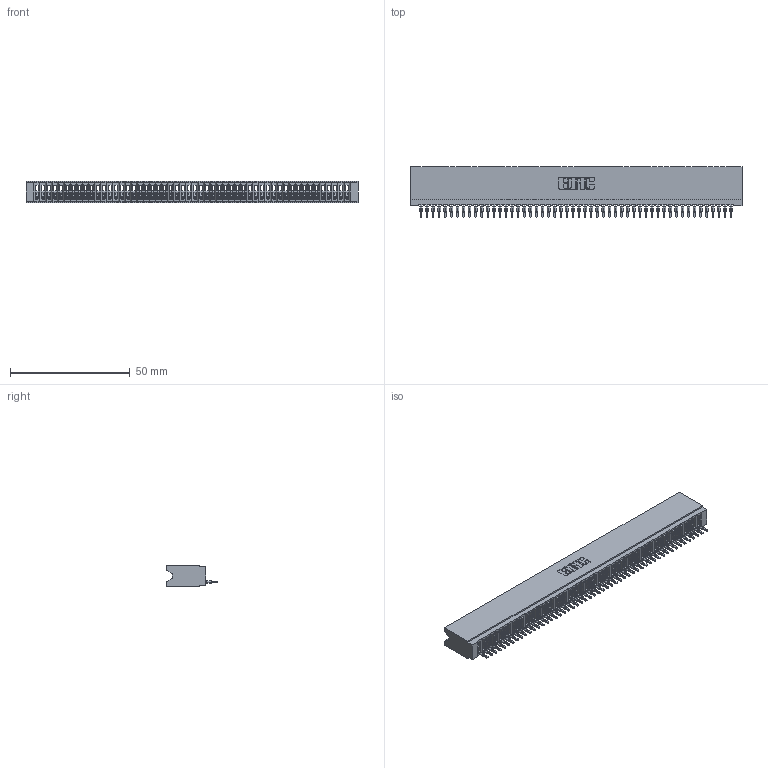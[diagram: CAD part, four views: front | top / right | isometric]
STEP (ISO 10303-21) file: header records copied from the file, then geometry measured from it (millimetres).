
FILE_DESCRIPTION (( 'STEP AP203' ), '1' );
FILE_NAME ('745-052-525-106.STEP', '2026-02-25T22:10:55', ( '' ), ( '' ), 'SwSTEP 2.0', 'SolidWorks 2023', '' );
FILE_SCHEMA (( 'CONFIG_CONTROL_DESIGN' ));
Length unit declared in the file: millimetre
Products named in the file (3): 745 Part_Insulator Option - 06; 745-292-001_525; 745-052-525-106
Assembly tree (53 placements, depth 2):
  745-052-525-106
    745 Part_Insulator Option - 06
    745-292-001_525  x52
Bounding box: 138.68 x 21.22 x 8.89 mm (x, y, z)
Volume: 11882.8 mm3; surface area: 22256.1 mm2
Topology: 53 solids, 53 shells, 5920 faces, 16276 edges, 10260 vertices
Faces by surface type: plane 3540, bspline 1040, cylinder 1028, torus 312
Entity records: 84534 total; most frequent: CARTESIAN_POINT 15398, ORIENTED_EDGE 14906, DIRECTION 12909, EDGE_CURVE 7453, LINE 6959, VECTOR 6959, VERTEX_POINT 4752, AXIS2_PLACEMENT_3D 2975
